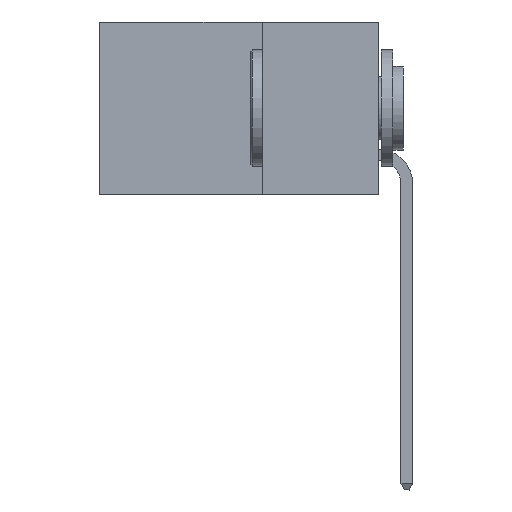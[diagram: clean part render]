
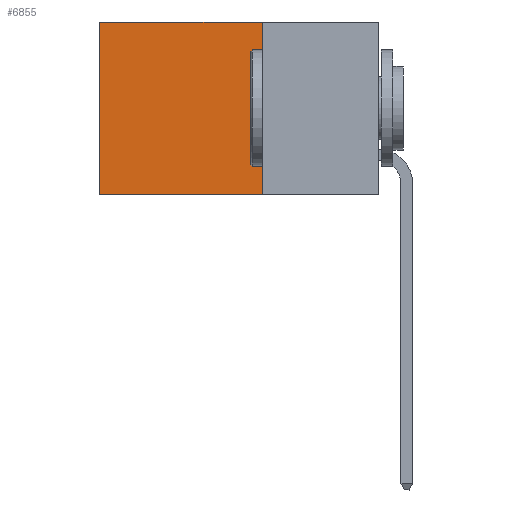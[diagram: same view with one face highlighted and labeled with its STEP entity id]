
A CAD part, left-side view. The second image highlights one B-rep face of the part: STEP entity #6855.
In plain terms, the highlighted planar face has unit normal (-1, 0, 0).
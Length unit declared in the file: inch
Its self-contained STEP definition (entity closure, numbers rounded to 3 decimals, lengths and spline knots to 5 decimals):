
#210 = CARTESIAN_POINT ( 'NONE',  ( 0.298, 0.25, 0. ) ) ;
#547 = CARTESIAN_POINT ( 'NONE',  ( 0.298, 0.25, 0. ) ) ;
#853 = VERTEX_POINT ( 'NONE', #6727 ) ;
#1616 = DIRECTION ( 'NONE',  ( 0., 0., -1. ) ) ;
#1847 = ORIENTED_EDGE ( 'NONE', *, *, #9305, .F. ) ;
#3132 = EDGE_CURVE ( 'NONE', #3719, #10674, #11518, .T. ) ;
#3719 = VERTEX_POINT ( 'NONE', #6305 ) ;
#4575 = CARTESIAN_POINT ( 'NONE',  ( 0.298, 0.6, -0.37 ) ) ;
#4625 = DIRECTION ( 'NONE',  ( 0., 1., 0. ) ) ;
#4792 = VECTOR ( 'NONE', #4625, 39.37008 ) ;
#5222 = LINE ( 'NONE', #16276, #4792 ) ;
#5266 = AXIS2_PLACEMENT_3D ( 'NONE', #13221, #13165, #12953 ) ;
#5677 = ORIENTED_EDGE ( 'NONE', *, *, #12610, .F. ) ;
#5814 = EDGE_LOOP ( 'NONE', ( #14749, #5677, #1847, #16183 ) ) ;
#6190 = VECTOR ( 'NONE', #16217, 39.37008 ) ;
#6305 = CARTESIAN_POINT ( 'NONE',  ( 0.298, 0.6, 0. ) ) ;
#6316 = VERTEX_POINT ( 'NONE', #547 ) ;
#6467 = EDGE_CURVE ( 'NONE', #6316, #3719, #5222, .T. ) ;
#6598 = VECTOR ( 'NONE', #1616, 39.37008 ) ;
#6727 = CARTESIAN_POINT ( 'NONE',  ( 0.298, 0.25, -0.37 ) ) ;
#6855 = ADVANCED_FACE ( 'NONE', ( #9237 ), #13300, .F. ) ;
#7017 = CARTESIAN_POINT ( 'NONE',  ( 0.298, 0.25, -0.37 ) ) ;
#8315 = LINE ( 'NONE', #7017, #6190 ) ;
#9237 = FACE_OUTER_BOUND ( 'NONE', #5814, .T. ) ;
#9305 = EDGE_CURVE ( 'NONE', #6316, #853, #17087, .T. ) ;
#10674 = VERTEX_POINT ( 'NONE', #4575 ) ;
#11518 = LINE ( 'NONE', #15997, #14516 ) ;
#12610 = EDGE_CURVE ( 'NONE', #853, #10674, #8315, .T. ) ;
#12953 = DIRECTION ( 'NONE',  ( 0., 0., -1. ) ) ;
#13165 = DIRECTION ( 'NONE',  ( 1., 0., 0. ) ) ;
#13221 = CARTESIAN_POINT ( 'NONE',  ( 0.298, 0.25, 0. ) ) ;
#13300 = PLANE ( 'NONE',  #5266 ) ;
#13829 = DIRECTION ( 'NONE',  ( 0., 0., -1. ) ) ;
#14516 = VECTOR ( 'NONE', #13829, 39.37008 ) ;
#14749 = ORIENTED_EDGE ( 'NONE', *, *, #3132, .T. ) ;
#15997 = CARTESIAN_POINT ( 'NONE',  ( 0.298, 0.6, 0. ) ) ;
#16183 = ORIENTED_EDGE ( 'NONE', *, *, #6467, .T. ) ;
#16217 = DIRECTION ( 'NONE',  ( 0., 1., 0. ) ) ;
#16276 = CARTESIAN_POINT ( 'NONE',  ( 0.298, 0.25, 0. ) ) ;
#17087 = LINE ( 'NONE', #210, #6598 ) ;
